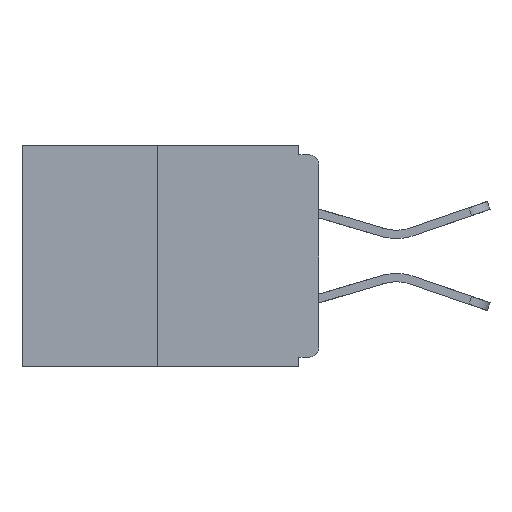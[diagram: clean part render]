
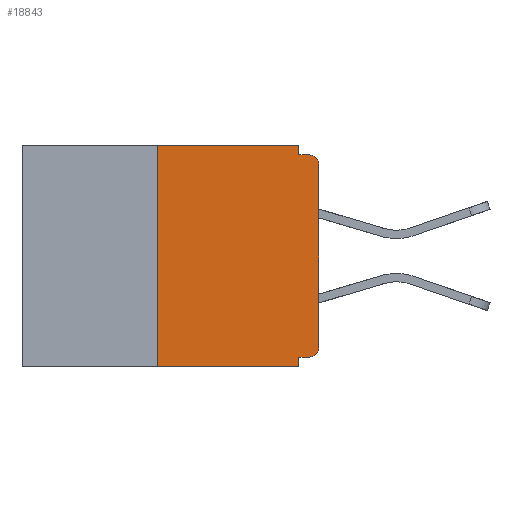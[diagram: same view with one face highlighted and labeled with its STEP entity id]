
A CAD part, left-side view. The second image highlights one B-rep face of the part: STEP entity #18843.
In plain terms, the highlighted planar face has unit normal (-1, 0, 0).
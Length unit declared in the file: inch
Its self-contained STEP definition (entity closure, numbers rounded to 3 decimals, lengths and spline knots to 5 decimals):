
#183 = LINE ( 'NONE', #4723, #23940 ) ;
#269 = EDGE_CURVE ( 'NONE', #3258, #9895, #183, .T. ) ;
#514 = PLANE ( 'NONE',  #24310 ) ;
#690 = ORIENTED_EDGE ( 'NONE', *, *, #4801, .F. ) ;
#757 = CARTESIAN_POINT ( 'NONE',  ( 0., 0.031, -0.328 ) ) ;
#764 = DIRECTION ( 'NONE',  ( -1., 0., 0. ) ) ;
#971 = CARTESIAN_POINT ( 'NONE',  ( 0., 0.015, -0.03 ) ) ;
#1113 = CIRCLE ( 'NONE', #6679, 0.015 ) ;
#1245 = DIRECTION ( 'NONE',  ( 0., 1., 0. ) ) ;
#1263 = DIRECTION ( 'NONE',  ( 0., 0., -1. ) ) ;
#1430 = CARTESIAN_POINT ( 'NONE',  ( 0., 0.25, -0.343 ) ) ;
#2102 = CARTESIAN_POINT ( 'NONE',  ( 0., 0.031, -0.015 ) ) ;
#2200 = AXIS2_PLACEMENT_3D ( 'NONE', #22607, #8152, #29770 ) ;
#2397 = VERTEX_POINT ( 'NONE', #26013 ) ;
#3232 = LINE ( 'NONE', #25014, #21052 ) ;
#3258 = VERTEX_POINT ( 'NONE', #1430 ) ;
#3329 = DIRECTION ( 'NONE',  ( 0., 0., -1. ) ) ;
#3587 = CARTESIAN_POINT ( 'NONE',  ( 0., 0., -0.015 ) ) ;
#4003 = DIRECTION ( 'NONE',  ( 0., 0., 1. ) ) ;
#4022 = CARTESIAN_POINT ( 'NONE',  ( 0., 0.25, 0. ) ) ;
#4723 = CARTESIAN_POINT ( 'NONE',  ( 0., 0.46, -0.343 ) ) ;
#4801 = EDGE_CURVE ( 'NONE', #22861, #17281, #23455, .T. ) ;
#5087 = EDGE_CURVE ( 'NONE', #15013, #16576, #5202, .T. ) ;
#5202 = LINE ( 'NONE', #19730, #11923 ) ;
#5651 = DIRECTION ( 'NONE',  ( 0., 0., -1. ) ) ;
#6679 = AXIS2_PLACEMENT_3D ( 'NONE', #971, #764, #3329 ) ;
#6797 = EDGE_CURVE ( 'NONE', #12373, #2397, #20255, .T. ) ;
#7008 = ORIENTED_EDGE ( 'NONE', *, *, #6797, .T. ) ;
#8152 = DIRECTION ( 'NONE',  ( -1., 0., 0. ) ) ;
#8414 = ORIENTED_EDGE ( 'NONE', *, *, #13240, .T. ) ;
#9895 = VERTEX_POINT ( 'NONE', #18513 ) ;
#10453 = CARTESIAN_POINT ( 'NONE',  ( 0., 0.015, -0.328 ) ) ;
#10884 = CARTESIAN_POINT ( 'NONE',  ( 0., 0., 0. ) ) ;
#11254 = ORIENTED_EDGE ( 'NONE', *, *, #28195, .T. ) ;
#11923 = VECTOR ( 'NONE', #12483, 39.37008 ) ;
#12092 = EDGE_CURVE ( 'NONE', #16576, #17614, #3232, .T. ) ;
#12373 = VERTEX_POINT ( 'NONE', #26277 ) ;
#12483 = DIRECTION ( 'NONE',  ( 0., -1., 0. ) ) ;
#13186 = VECTOR ( 'NONE', #4003, 39.37008 ) ;
#13240 = EDGE_CURVE ( 'NONE', #2397, #28310, #1113, .T. ) ;
#14634 = LINE ( 'NONE', #3587, #28003 ) ;
#14703 = CARTESIAN_POINT ( 'NONE',  ( 0., 0.46, 0. ) ) ;
#14942 = ORIENTED_EDGE ( 'NONE', *, *, #5087, .F. ) ;
#15005 = DIRECTION ( 'NONE',  ( 1., 0., 0. ) ) ;
#15013 = VERTEX_POINT ( 'NONE', #16508 ) ;
#15438 = CARTESIAN_POINT ( 'NONE',  ( 0., 0., -0.328 ) ) ;
#16280 = EDGE_CURVE ( 'NONE', #17281, #9895, #26786, .T. ) ;
#16508 = CARTESIAN_POINT ( 'NONE',  ( 0., 0.25, 0. ) ) ;
#16576 = VERTEX_POINT ( 'NONE', #24374 ) ;
#17281 = VERTEX_POINT ( 'NONE', #757 ) ;
#17387 = CARTESIAN_POINT ( 'NONE',  ( 0., 0.015, -0.015 ) ) ;
#17614 = VERTEX_POINT ( 'NONE', #2102 ) ;
#18387 = EDGE_CURVE ( 'NONE', #3258, #15013, #25151, .T. ) ;
#18513 = CARTESIAN_POINT ( 'NONE',  ( 0., 0.031, -0.343 ) ) ;
#18826 = VECTOR ( 'NONE', #21243, 39.37008 ) ;
#18843 = ADVANCED_FACE ( 'NONE', ( #20677 ), #514, .F. ) ;
#19333 = ORIENTED_EDGE ( 'NONE', *, *, #12092, .F. ) ;
#19730 = CARTESIAN_POINT ( 'NONE',  ( 0., 0.46, 0. ) ) ;
#20255 = LINE ( 'NONE', #10884, #13186 ) ;
#20307 = EDGE_LOOP ( 'NONE', ( #14942, #30009, #22769, #29260, #690, #11254, #7008, #8414, #27904, #19333 ) ) ;
#20677 = FACE_OUTER_BOUND ( 'NONE', #20307, .T. ) ;
#21052 = VECTOR ( 'NONE', #1263, 39.37008 ) ;
#21243 = DIRECTION ( 'NONE',  ( 0., 0., 1. ) ) ;
#22607 = CARTESIAN_POINT ( 'NONE',  ( 0., 0.015, -0.313 ) ) ;
#22769 = ORIENTED_EDGE ( 'NONE', *, *, #269, .T. ) ;
#22861 = VERTEX_POINT ( 'NONE', #10453 ) ;
#22904 = DIRECTION ( 'NONE',  ( 0., -1., 0. ) ) ;
#23455 = LINE ( 'NONE', #15438, #24202 ) ;
#23940 = VECTOR ( 'NONE', #25838, 39.37008 ) ;
#24153 = EDGE_CURVE ( 'NONE', #17614, #28310, #14634, .T. ) ;
#24202 = VECTOR ( 'NONE', #1245, 39.37008 ) ;
#24310 = AXIS2_PLACEMENT_3D ( 'NONE', #14703, #15005, #5651 ) ;
#24374 = CARTESIAN_POINT ( 'NONE',  ( 0., 0.031, 0. ) ) ;
#25014 = CARTESIAN_POINT ( 'NONE',  ( 0., 0.031, 0. ) ) ;
#25151 = LINE ( 'NONE', #4022, #18826 ) ;
#25678 = VECTOR ( 'NONE', #30236, 39.37008 ) ;
#25838 = DIRECTION ( 'NONE',  ( 0., -1., 0. ) ) ;
#26013 = CARTESIAN_POINT ( 'NONE',  ( 0., 0., -0.03 ) ) ;
#26277 = CARTESIAN_POINT ( 'NONE',  ( 0., 0., -0.313 ) ) ;
#26786 = LINE ( 'NONE', #29519, #25678 ) ;
#27904 = ORIENTED_EDGE ( 'NONE', *, *, #24153, .F. ) ;
#28003 = VECTOR ( 'NONE', #22904, 39.37008 ) ;
#28195 = EDGE_CURVE ( 'NONE', #22861, #12373, #29781, .T. ) ;
#28310 = VERTEX_POINT ( 'NONE', #17387 ) ;
#29260 = ORIENTED_EDGE ( 'NONE', *, *, #16280, .F. ) ;
#29519 = CARTESIAN_POINT ( 'NONE',  ( 0., 0.031, -0.343 ) ) ;
#29770 = DIRECTION ( 'NONE',  ( 0., 0., -1. ) ) ;
#29781 = CIRCLE ( 'NONE', #2200, 0.015 ) ;
#30009 = ORIENTED_EDGE ( 'NONE', *, *, #18387, .F. ) ;
#30236 = DIRECTION ( 'NONE',  ( 0., 0., -1. ) ) ;
